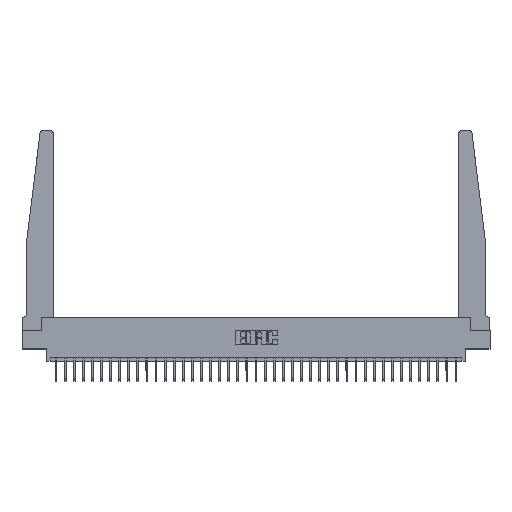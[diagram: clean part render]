
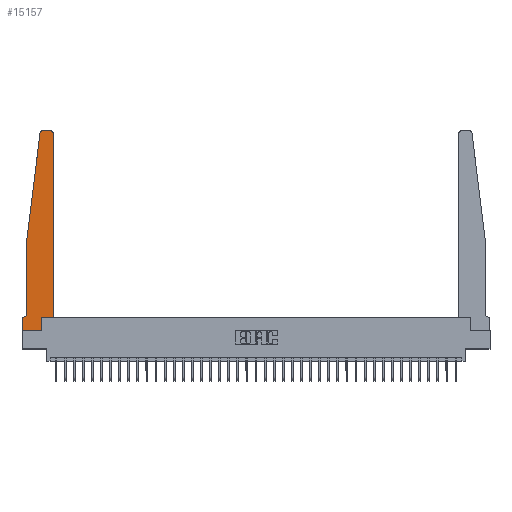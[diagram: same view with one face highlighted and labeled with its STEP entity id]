
A CAD part, top view. The second image highlights one B-rep face of the part: STEP entity #15157.
In plain terms, the highlighted planar face has unit normal (0, 0, 1).
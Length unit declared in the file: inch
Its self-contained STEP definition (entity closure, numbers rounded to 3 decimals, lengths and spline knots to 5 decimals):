
#304 = VERTEX_POINT ( 'NONE', #24170 ) ;
#589 = LINE ( 'NONE', #13473, #25949 ) ;
#982 = DIRECTION ( 'NONE',  ( 0., 0., -1. ) ) ;
#1095 = CARTESIAN_POINT ( 'NONE',  ( 0.425, 0.18, 0.37 ) ) ;
#1239 = CARTESIAN_POINT ( 'NONE',  ( 0.2605, 0.18, 0.37 ) ) ;
#1679 = ORIENTED_EDGE ( 'NONE', *, *, #29608, .T. ) ;
#2012 = CARTESIAN_POINT ( 'NONE',  ( 0.25, 2.75, 0.37 ) ) ;
#2111 = VECTOR ( 'NONE', #12519, 39.37008 ) ;
#3624 = DIRECTION ( 'NONE',  ( -1., 0., 0. ) ) ;
#3751 = CARTESIAN_POINT ( 'NONE',  ( 0.2605, 0., 0.37 ) ) ;
#3862 = DIRECTION ( 'NONE',  ( 0., 0., 1. ) ) ;
#3887 = VERTEX_POINT ( 'NONE', #3751 ) ;
#4712 = ORIENTED_EDGE ( 'NONE', *, *, #15023, .T. ) ;
#4862 = ORIENTED_EDGE ( 'NONE', *, *, #12980, .T. ) ;
#5475 = EDGE_CURVE ( 'NONE', #34689, #3887, #5708, .T. ) ;
#5697 = ORIENTED_EDGE ( 'NONE', *, *, #29775, .T. ) ;
#5708 = LINE ( 'NONE', #10273, #30298 ) ;
#6183 = DIRECTION ( 'NONE',  ( 1., 0., 0. ) ) ;
#6239 = CARTESIAN_POINT ( 'NONE',  ( 0.425, 2.72, 0.37 ) ) ;
#7080 = CARTESIAN_POINT ( 'NONE',  ( 0.24675, 2.72367, 0.37 ) ) ;
#7186 = DIRECTION ( 'NONE',  ( 1., 0., 0. ) ) ;
#7434 = DIRECTION ( 'NONE',  ( 1., 0., 0. ) ) ;
#7509 = EDGE_CURVE ( 'NONE', #7780, #11275, #32781, .T. ) ;
#7780 = VERTEX_POINT ( 'NONE', #10351 ) ;
#8147 = CARTESIAN_POINT ( 'NONE',  ( 0., 0., 0.37 ) ) ;
#8643 = VERTEX_POINT ( 'NONE', #22766 ) ;
#8839 = EDGE_LOOP ( 'NONE', ( #13490, #4712, #34818, #30540, #11147, #21568, #33912, #10634, #30453, #4862, #1679, #5697 ) ) ;
#9082 = EDGE_CURVE ( 'NONE', #9164, #8643, #30019, .T. ) ;
#9164 = VERTEX_POINT ( 'NONE', #28709 ) ;
#9386 = CIRCLE ( 'NONE', #21142, 0.05 ) ;
#9776 = DIRECTION ( 'NONE',  ( 0., -1., 0. ) ) ;
#9984 = DIRECTION ( 'NONE',  ( 0., 0., 1. ) ) ;
#10055 = VERTEX_POINT ( 'NONE', #6239 ) ;
#10210 = DIRECTION ( 'NONE',  ( 0., 1., 0. ) ) ;
#10273 = CARTESIAN_POINT ( 'NONE',  ( 0., 0., 0.37 ) ) ;
#10351 = CARTESIAN_POINT ( 'NONE',  ( 0.015, 0.1875, 0.37 ) ) ;
#10532 = CARTESIAN_POINT ( 'NONE',  ( 0., 0.1875, 0.37 ) ) ;
#10634 = ORIENTED_EDGE ( 'NONE', *, *, #5475, .T. ) ;
#11147 = ORIENTED_EDGE ( 'NONE', *, *, #28415, .T. ) ;
#11275 = VERTEX_POINT ( 'NONE', #10532 ) ;
#12004 = DIRECTION ( 'NONE',  ( 1., 0., 0. ) ) ;
#12277 = CARTESIAN_POINT ( 'NONE',  ( 0.065, 1.25, 0.37 ) ) ;
#12519 = DIRECTION ( 'NONE',  ( 0., 1., 0. ) ) ;
#12739 = CARTESIAN_POINT ( 'NONE',  ( 0.065, 0.1875, 0.37 ) ) ;
#12842 = PLANE ( 'NONE',  #29913 ) ;
#12980 = EDGE_CURVE ( 'NONE', #23959, #304, #35159, .T. ) ;
#13034 = LINE ( 'NONE', #14457, #25528 ) ;
#13473 = CARTESIAN_POINT ( 'NONE',  ( 0.065, 1.25, 0.37 ) ) ;
#13490 = ORIENTED_EDGE ( 'NONE', *, *, #9082, .T. ) ;
#13535 = AXIS2_PLACEMENT_3D ( 'NONE', #13546, #27373, #6183 ) ;
#13546 = CARTESIAN_POINT ( 'NONE',  ( 0.395, 2.72, 0.37 ) ) ;
#14457 = CARTESIAN_POINT ( 'NONE',  ( 0., 0., 0.37 ) ) ;
#15023 = EDGE_CURVE ( 'NONE', #8643, #15741, #31980, .T. ) ;
#15157 = ADVANCED_FACE ( 'NONE', ( #30613 ), #12842, .T. ) ;
#15741 = VERTEX_POINT ( 'NONE', #7080 ) ;
#16529 = VECTOR ( 'NONE', #7186, 39.37008 ) ;
#16629 = CARTESIAN_POINT ( 'NONE',  ( 0.065, 1.25, 0.37 ) ) ;
#18037 = VECTOR ( 'NONE', #29260, 39.37008 ) ;
#18068 = CARTESIAN_POINT ( 'NONE',  ( 0.065, 0.2375, 0.37 ) ) ;
#18251 = CIRCLE ( 'NONE', #13535, 0.03 ) ;
#18520 = DIRECTION ( 'NONE',  ( 1., 0., 0. ) ) ;
#18843 = VERTEX_POINT ( 'NONE', #16629 ) ;
#19043 = VECTOR ( 'NONE', #9776, 39.37008 ) ;
#19676 = CARTESIAN_POINT ( 'NONE',  ( 0.015, 0.2375, 0.37 ) ) ;
#20429 = VERTEX_POINT ( 'NONE', #18068 ) ;
#20643 = EDGE_CURVE ( 'NONE', #3887, #23959, #29638, .T. ) ;
#21142 = AXIS2_PLACEMENT_3D ( 'NONE', #19676, #982, #3624 ) ;
#21351 = LINE ( 'NONE', #26685, #34330 ) ;
#21568 = ORIENTED_EDGE ( 'NONE', *, *, #7509, .T. ) ;
#22766 = CARTESIAN_POINT ( 'NONE',  ( 0.27653, 2.75, 0.37 ) ) ;
#22959 = LINE ( 'NONE', #12277, #19043 ) ;
#23140 = DIRECTION ( 'NONE',  ( 0., -1., 0. ) ) ;
#23315 = EDGE_CURVE ( 'NONE', #11275, #34689, #13034, .T. ) ;
#23959 = VERTEX_POINT ( 'NONE', #1239 ) ;
#24170 = CARTESIAN_POINT ( 'NONE',  ( 0.425, 0.18, 0.37 ) ) ;
#25528 = VECTOR ( 'NONE', #23140, 39.37008 ) ;
#25949 = VECTOR ( 'NONE', #26484, 39.37008 ) ;
#26484 = DIRECTION ( 'NONE',  ( -0.122, -0.992, 0. ) ) ;
#26685 = CARTESIAN_POINT ( 'NONE',  ( 0.425, 0.18, 0.37 ) ) ;
#27373 = DIRECTION ( 'NONE',  ( 0., 0., 1. ) ) ;
#28415 = EDGE_CURVE ( 'NONE', #20429, #7780, #9386, .T. ) ;
#28484 = CARTESIAN_POINT ( 'NONE',  ( 0.27653, 2.72, 0.37 ) ) ;
#28503 = DIRECTION ( 'NONE',  ( -1., 0., 0. ) ) ;
#28709 = CARTESIAN_POINT ( 'NONE',  ( 0.395, 2.75, 0.37 ) ) ;
#29260 = DIRECTION ( 'NONE',  ( -1., 0., 0. ) ) ;
#29608 = EDGE_CURVE ( 'NONE', #304, #10055, #21351, .T. ) ;
#29638 = LINE ( 'NONE', #34983, #2111 ) ;
#29775 = EDGE_CURVE ( 'NONE', #10055, #9164, #18251, .T. ) ;
#29913 = AXIS2_PLACEMENT_3D ( 'NONE', #32174, #9984, #7434 ) ;
#30019 = LINE ( 'NONE', #2012, #34392 ) ;
#30298 = VECTOR ( 'NONE', #18520, 39.37008 ) ;
#30453 = ORIENTED_EDGE ( 'NONE', *, *, #20643, .T. ) ;
#30540 = ORIENTED_EDGE ( 'NONE', *, *, #30719, .T. ) ;
#30613 = FACE_OUTER_BOUND ( 'NONE', #8839, .T. ) ;
#30719 = EDGE_CURVE ( 'NONE', #18843, #20429, #22959, .T. ) ;
#30876 = EDGE_CURVE ( 'NONE', #15741, #18843, #589, .T. ) ;
#31980 = CIRCLE ( 'NONE', #33645, 0.03 ) ;
#32174 = CARTESIAN_POINT ( 'NONE',  ( 0., 0.1875, 0.37 ) ) ;
#32781 = LINE ( 'NONE', #12739, #18037 ) ;
#33645 = AXIS2_PLACEMENT_3D ( 'NONE', #28484, #3862, #12004 ) ;
#33912 = ORIENTED_EDGE ( 'NONE', *, *, #23315, .T. ) ;
#34330 = VECTOR ( 'NONE', #10210, 39.37008 ) ;
#34392 = VECTOR ( 'NONE', #28503, 39.37008 ) ;
#34689 = VERTEX_POINT ( 'NONE', #8147 ) ;
#34818 = ORIENTED_EDGE ( 'NONE', *, *, #30876, .T. ) ;
#34983 = CARTESIAN_POINT ( 'NONE',  ( 0.2605, 0.18, 0.37 ) ) ;
#35159 = LINE ( 'NONE', #1095, #16529 ) ;
